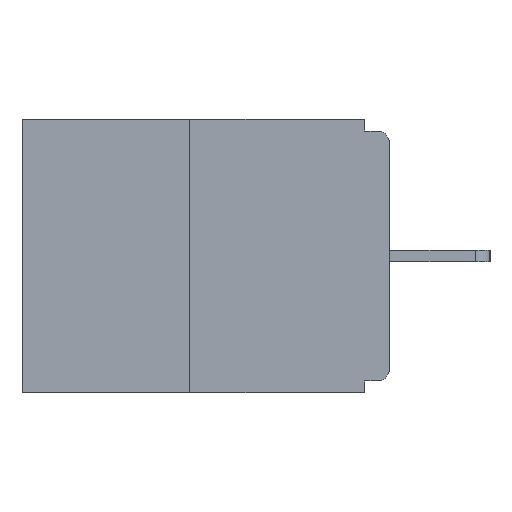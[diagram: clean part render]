
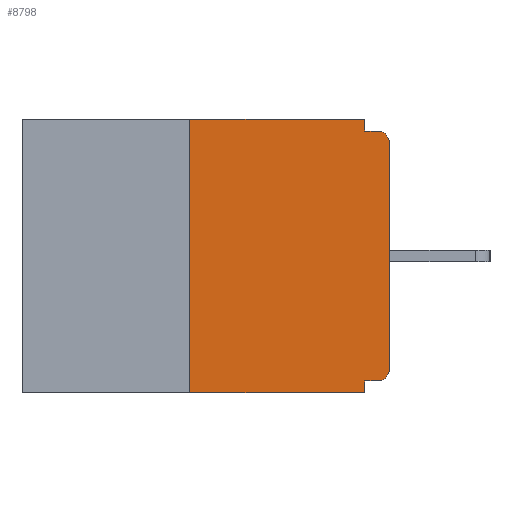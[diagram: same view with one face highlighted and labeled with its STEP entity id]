
A CAD part, left-side view. The second image highlights one B-rep face of the part: STEP entity #8798.
In plain terms, the highlighted planar face has unit normal (-1, 0, 0).
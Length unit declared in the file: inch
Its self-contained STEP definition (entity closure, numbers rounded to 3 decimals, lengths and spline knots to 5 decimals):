
#73 = ORIENTED_EDGE ( 'NONE', *, *, #23795, .F. ) ;
#227 = CARTESIAN_POINT ( 'NONE',  ( 0., 0.46, -0.343 ) ) ;
#277 = DIRECTION ( 'NONE',  ( 0., 0., -1. ) ) ;
#666 = VERTEX_POINT ( 'NONE', #11510 ) ;
#952 = CARTESIAN_POINT ( 'NONE',  ( 0., 0., -0.313 ) ) ;
#1141 = EDGE_CURVE ( 'NONE', #13617, #666, #13286, .T. ) ;
#1853 = LINE ( 'NONE', #15104, #6517 ) ;
#2543 = LINE ( 'NONE', #13892, #11724 ) ;
#2655 = DIRECTION ( 'NONE',  ( 0., 1., 0. ) ) ;
#3191 = AXIS2_PLACEMENT_3D ( 'NONE', #19022, #18850, #18777 ) ;
#3199 = ORIENTED_EDGE ( 'NONE', *, *, #18914, .T. ) ;
#3373 = CARTESIAN_POINT ( 'NONE',  ( 0., 0.015, -0.313 ) ) ;
#3544 = CARTESIAN_POINT ( 'NONE',  ( 0., 0.031, -0.015 ) ) ;
#4120 = LINE ( 'NONE', #21600, #14407 ) ;
#4199 = AXIS2_PLACEMENT_3D ( 'NONE', #3373, #16880, #5359 ) ;
#4666 = EDGE_CURVE ( 'NONE', #18808, #18356, #4120, .T. ) ;
#5359 = DIRECTION ( 'NONE',  ( 0., 0., -1. ) ) ;
#5617 = VERTEX_POINT ( 'NONE', #16748 ) ;
#6233 = ORIENTED_EDGE ( 'NONE', *, *, #1141, .F. ) ;
#6443 = CARTESIAN_POINT ( 'NONE',  ( 0., 0., -0.015 ) ) ;
#6517 = VECTOR ( 'NONE', #17037, 39.37008 ) ;
#7006 = CIRCLE ( 'NONE', #4199, 0.015 ) ;
#7156 = LINE ( 'NONE', #12395, #12259 ) ;
#7243 = EDGE_CURVE ( 'NONE', #18356, #10584, #8360, .T. ) ;
#7507 = CARTESIAN_POINT ( 'NONE',  ( 0., 0.25, 0. ) ) ;
#7823 = CARTESIAN_POINT ( 'NONE',  ( 0., 0.46, 0. ) ) ;
#7924 = VECTOR ( 'NONE', #23696, 39.37008 ) ;
#8106 = VERTEX_POINT ( 'NONE', #3544 ) ;
#8245 = VECTOR ( 'NONE', #19630, 39.37008 ) ;
#8282 = CARTESIAN_POINT ( 'NONE',  ( 0., 0.031, -0.328 ) ) ;
#8299 = DIRECTION ( 'NONE',  ( 0., -1., 0. ) ) ;
#8360 = CIRCLE ( 'NONE', #3191, 0.015 ) ;
#8798 = ADVANCED_FACE ( 'NONE', ( #22900 ), #24905, .F. ) ;
#9425 = EDGE_CURVE ( 'NONE', #13226, #666, #14517, .T. ) ;
#9550 = ORIENTED_EDGE ( 'NONE', *, *, #19514, .F. ) ;
#9769 = DIRECTION ( 'NONE',  ( 0., 0., -1. ) ) ;
#10355 = ORIENTED_EDGE ( 'NONE', *, *, #23226, .F. ) ;
#10584 = VERTEX_POINT ( 'NONE', #11723 ) ;
#11276 = CARTESIAN_POINT ( 'NONE',  ( 0., 0., -0.03 ) ) ;
#11510 = CARTESIAN_POINT ( 'NONE',  ( 0., 0.031, -0.343 ) ) ;
#11723 = CARTESIAN_POINT ( 'NONE',  ( 0., 0.015, -0.015 ) ) ;
#11724 = VECTOR ( 'NONE', #277, 39.37008 ) ;
#11731 = VERTEX_POINT ( 'NONE', #19330 ) ;
#11843 = EDGE_CURVE ( 'NONE', #5617, #8106, #2543, .T. ) ;
#12191 = CARTESIAN_POINT ( 'NONE',  ( 0., 0.25, -0.343 ) ) ;
#12259 = VECTOR ( 'NONE', #2655, 39.37008 ) ;
#12395 = CARTESIAN_POINT ( 'NONE',  ( 0., 0., -0.328 ) ) ;
#13226 = VERTEX_POINT ( 'NONE', #12191 ) ;
#13286 = LINE ( 'NONE', #18942, #8245 ) ;
#13463 = VECTOR ( 'NONE', #14145, 39.37008 ) ;
#13617 = VERTEX_POINT ( 'NONE', #8282 ) ;
#13892 = CARTESIAN_POINT ( 'NONE',  ( 0., 0.031, 0. ) ) ;
#14054 = LINE ( 'NONE', #23690, #13463 ) ;
#14145 = DIRECTION ( 'NONE',  ( 0., 0., 1. ) ) ;
#14407 = VECTOR ( 'NONE', #21624, 39.37008 ) ;
#14517 = LINE ( 'NONE', #227, #19010 ) ;
#15104 = CARTESIAN_POINT ( 'NONE',  ( 0., 0.46, 0. ) ) ;
#15727 = EDGE_CURVE ( 'NONE', #16542, #5617, #1853, .T. ) ;
#16343 = ORIENTED_EDGE ( 'NONE', *, *, #15727, .F. ) ;
#16542 = VERTEX_POINT ( 'NONE', #7507 ) ;
#16748 = CARTESIAN_POINT ( 'NONE',  ( 0., 0.031, 0. ) ) ;
#16880 = DIRECTION ( 'NONE',  ( -1., 0., 0. ) ) ;
#17037 = DIRECTION ( 'NONE',  ( 0., -1., 0. ) ) ;
#18302 = ORIENTED_EDGE ( 'NONE', *, *, #4666, .T. ) ;
#18356 = VERTEX_POINT ( 'NONE', #11276 ) ;
#18441 = ORIENTED_EDGE ( 'NONE', *, *, #7243, .T. ) ;
#18555 = AXIS2_PLACEMENT_3D ( 'NONE', #7823, #21174, #9769 ) ;
#18777 = DIRECTION ( 'NONE',  ( 0., 0., -1. ) ) ;
#18808 = VERTEX_POINT ( 'NONE', #952 ) ;
#18850 = DIRECTION ( 'NONE',  ( -1., 0., 0. ) ) ;
#18914 = EDGE_CURVE ( 'NONE', #11731, #18808, #7006, .T. ) ;
#18942 = CARTESIAN_POINT ( 'NONE',  ( 0., 0.031, -0.343 ) ) ;
#19010 = VECTOR ( 'NONE', #8299, 39.37008 ) ;
#19022 = CARTESIAN_POINT ( 'NONE',  ( 0., 0.015, -0.03 ) ) ;
#19094 = ORIENTED_EDGE ( 'NONE', *, *, #11843, .F. ) ;
#19330 = CARTESIAN_POINT ( 'NONE',  ( 0., 0.015, -0.328 ) ) ;
#19514 = EDGE_CURVE ( 'NONE', #8106, #10584, #23144, .T. ) ;
#19630 = DIRECTION ( 'NONE',  ( 0., 0., -1. ) ) ;
#20618 = ORIENTED_EDGE ( 'NONE', *, *, #9425, .T. ) ;
#21174 = DIRECTION ( 'NONE',  ( 1., 0., 0. ) ) ;
#21600 = CARTESIAN_POINT ( 'NONE',  ( 0., 0., 0. ) ) ;
#21624 = DIRECTION ( 'NONE',  ( 0., 0., 1. ) ) ;
#22900 = FACE_OUTER_BOUND ( 'NONE', #24675, .T. ) ;
#23144 = LINE ( 'NONE', #6443, #7924 ) ;
#23226 = EDGE_CURVE ( 'NONE', #13226, #16542, #14054, .T. ) ;
#23690 = CARTESIAN_POINT ( 'NONE',  ( 0., 0.25, 0. ) ) ;
#23696 = DIRECTION ( 'NONE',  ( 0., -1., 0. ) ) ;
#23795 = EDGE_CURVE ( 'NONE', #11731, #13617, #7156, .T. ) ;
#24675 = EDGE_LOOP ( 'NONE', ( #16343, #10355, #20618, #6233, #73, #3199, #18302, #18441, #9550, #19094 ) ) ;
#24905 = PLANE ( 'NONE',  #18555 ) ;
